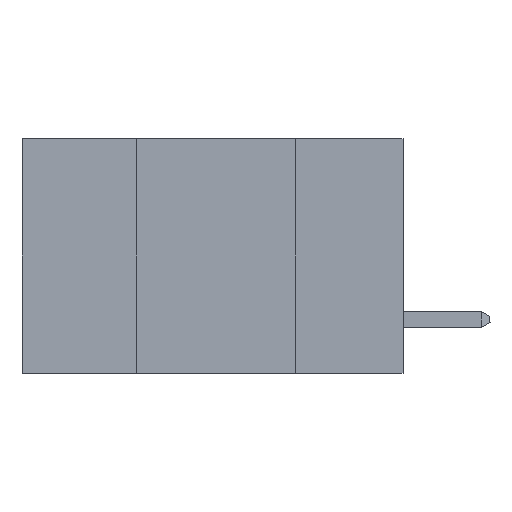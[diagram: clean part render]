
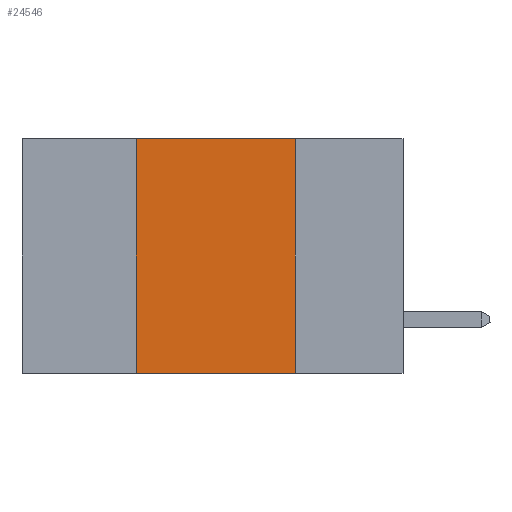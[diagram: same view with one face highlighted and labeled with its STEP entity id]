
A CAD part, left-side view. The second image highlights one B-rep face of the part: STEP entity #24546.
In plain terms, the highlighted planar face has unit normal (-1, 0, 0).
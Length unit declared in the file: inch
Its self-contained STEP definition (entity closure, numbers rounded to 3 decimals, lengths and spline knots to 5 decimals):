
#1183 = CARTESIAN_POINT ( 'NONE',  ( 0., 0.42, 0. ) ) ;
#1873 = ORIENTED_EDGE ( 'NONE', *, *, #4553, .F. ) ;
#1943 = CARTESIAN_POINT ( 'NONE',  ( 0., 0.17, -0.37 ) ) ;
#2444 = CARTESIAN_POINT ( 'NONE',  ( 0., 0.42, 0. ) ) ;
#3493 = CARTESIAN_POINT ( 'NONE',  ( 0., 0.6, -0.37 ) ) ;
#3922 = CARTESIAN_POINT ( 'NONE',  ( 0., 0.6, 0. ) ) ;
#4553 = EDGE_CURVE ( 'NONE', #26813, #32124, #25016, .T. ) ;
#5232 = LINE ( 'NONE', #2444, #23114 ) ;
#5268 = DIRECTION ( 'NONE',  ( 0., 0., 1. ) ) ;
#6049 = CARTESIAN_POINT ( 'NONE',  ( 0., 0.6, 0. ) ) ;
#6346 = VECTOR ( 'NONE', #24760, 39.37008 ) ;
#6401 = CARTESIAN_POINT ( 'NONE',  ( 0., 0.42, -0.37 ) ) ;
#6684 = PLANE ( 'NONE',  #14964 ) ;
#7264 = EDGE_LOOP ( 'NONE', ( #1873, #25788, #13912, #32887 ) ) ;
#8532 = DIRECTION ( 'NONE',  ( 0., -1., 0. ) ) ;
#10673 = VERTEX_POINT ( 'NONE', #6401 ) ;
#11258 = EDGE_CURVE ( 'NONE', #10673, #32124, #30105, .T. ) ;
#11703 = DIRECTION ( 'NONE',  ( 1., 0., 0. ) ) ;
#11723 = EDGE_CURVE ( 'NONE', #10673, #12491, #5232, .T. ) ;
#12491 = VERTEX_POINT ( 'NONE', #1183 ) ;
#13200 = EDGE_CURVE ( 'NONE', #12491, #26813, #21276, .T. ) ;
#13912 = ORIENTED_EDGE ( 'NONE', *, *, #11723, .F. ) ;
#14964 = AXIS2_PLACEMENT_3D ( 'NONE', #3922, #11703, #30283 ) ;
#15295 = CARTESIAN_POINT ( 'NONE',  ( 0., 0.17, 0. ) ) ;
#19587 = VECTOR ( 'NONE', #31584, 39.37008 ) ;
#21276 = LINE ( 'NONE', #6049, #6346 ) ;
#23114 = VECTOR ( 'NONE', #5268, 39.37008 ) ;
#24546 = ADVANCED_FACE ( 'NONE', ( #31879 ), #6684, .F. ) ;
#24760 = DIRECTION ( 'NONE',  ( 0., -1., 0. ) ) ;
#25016 = LINE ( 'NONE', #26796, #19587 ) ;
#25788 = ORIENTED_EDGE ( 'NONE', *, *, #13200, .F. ) ;
#26796 = CARTESIAN_POINT ( 'NONE',  ( 0., 0.17, 0. ) ) ;
#26813 = VERTEX_POINT ( 'NONE', #15295 ) ;
#30105 = LINE ( 'NONE', #3493, #30533 ) ;
#30283 = DIRECTION ( 'NONE',  ( 0., 0., -1. ) ) ;
#30533 = VECTOR ( 'NONE', #8532, 39.37008 ) ;
#31584 = DIRECTION ( 'NONE',  ( 0., 0., -1. ) ) ;
#31879 = FACE_OUTER_BOUND ( 'NONE', #7264, .T. ) ;
#32124 = VERTEX_POINT ( 'NONE', #1943 ) ;
#32887 = ORIENTED_EDGE ( 'NONE', *, *, #11258, .T. ) ;
